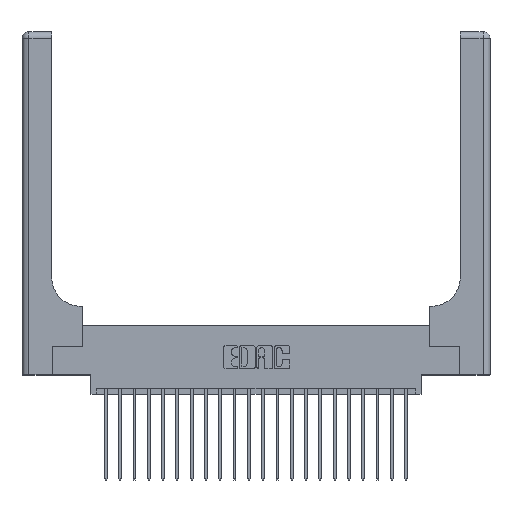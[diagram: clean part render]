
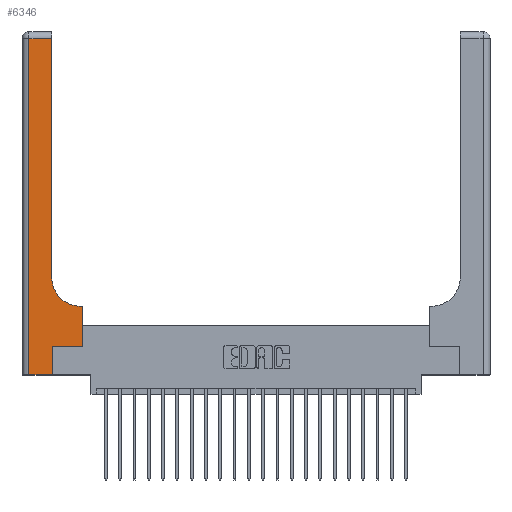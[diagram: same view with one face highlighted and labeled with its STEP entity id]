
A CAD part, top view. The second image highlights one B-rep face of the part: STEP entity #6346.
In plain terms, the highlighted planar face has unit normal (0, 0, 1).
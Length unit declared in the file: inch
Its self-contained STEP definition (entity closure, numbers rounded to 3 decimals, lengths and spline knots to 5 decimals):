
#209 = ORIENTED_EDGE ( 'NONE', *, *, #18631, .T. ) ;
#318 = CARTESIAN_POINT ( 'NONE',  ( 0.528, 0.6, 0.37 ) ) ;
#325 = VECTOR ( 'NONE', #9154, 39.37008 ) ;
#718 = CARTESIAN_POINT ( 'NONE',  ( 0., 3., 0.37 ) ) ;
#719 = ORIENTED_EDGE ( 'NONE', *, *, #10867, .T. ) ;
#832 = FACE_OUTER_BOUND ( 'NONE', #22626, .T. ) ;
#1018 = ORIENTED_EDGE ( 'NONE', *, *, #12879, .T. ) ;
#1352 = CARTESIAN_POINT ( 'NONE',  ( 0.265, 0.25, 0.37 ) ) ;
#1356 = LINE ( 'NONE', #21672, #8314 ) ;
#1602 = DIRECTION ( 'NONE',  ( 0., 1., 0. ) ) ;
#2286 = CARTESIAN_POINT ( 'NONE',  ( 0.528, 0.25, 0.37 ) ) ;
#2618 = VERTEX_POINT ( 'NONE', #15560 ) ;
#3192 = DIRECTION ( 'NONE',  ( 1., 0., 0. ) ) ;
#3220 = VECTOR ( 'NONE', #3192, 39.37008 ) ;
#3402 = DIRECTION ( 'NONE',  ( -1., 0., 0. ) ) ;
#3409 = VERTEX_POINT ( 'NONE', #13255 ) ;
#3488 = VERTEX_POINT ( 'NONE', #17016 ) ;
#3734 = VERTEX_POINT ( 'NONE', #8714 ) ;
#4235 = LINE ( 'NONE', #2286, #4493 ) ;
#4315 = CARTESIAN_POINT ( 'NONE',  ( 0., 0., 0.37 ) ) ;
#4481 = EDGE_CURVE ( 'NONE', #2618, #10803, #20533, .T. ) ;
#4493 = VECTOR ( 'NONE', #19701, 39.37008 ) ;
#4520 = VERTEX_POINT ( 'NONE', #17272 ) ;
#5045 = VECTOR ( 'NONE', #1602, 39.37008 ) ;
#5524 = EDGE_CURVE ( 'NONE', #3734, #18050, #4235, .T. ) ;
#6096 = VERTEX_POINT ( 'NONE', #16983 ) ;
#6346 = ADVANCED_FACE ( 'NONE', ( #832 ), #22198, .F. ) ;
#6915 = ORIENTED_EDGE ( 'NONE', *, *, #20098, .T. ) ;
#8314 = VECTOR ( 'NONE', #8965, 39.37008 ) ;
#8714 = CARTESIAN_POINT ( 'NONE',  ( 0.528, 0.25, 0.37 ) ) ;
#8965 = DIRECTION ( 'NONE',  ( -1., 0., 0. ) ) ;
#9154 = DIRECTION ( 'NONE',  ( 0., 1., 0. ) ) ;
#9383 = DIRECTION ( 'NONE',  ( 1., 0., 0. ) ) ;
#10392 = DIRECTION ( 'NONE',  ( 0., -1., 0. ) ) ;
#10803 = VERTEX_POINT ( 'NONE', #1352 ) ;
#10851 = CARTESIAN_POINT ( 'NONE',  ( 0.51, 0.6, 0.37 ) ) ;
#10867 = EDGE_CURVE ( 'NONE', #16644, #6096, #11961, .T. ) ;
#11488 = ORIENTED_EDGE ( 'NONE', *, *, #14473, .T. ) ;
#11646 = CARTESIAN_POINT ( 'NONE',  ( 0.265, 0., 0.37 ) ) ;
#11955 = LINE ( 'NONE', #18976, #3220 ) ;
#11961 = CIRCLE ( 'NONE', #13434, 0.25 ) ;
#12879 = EDGE_CURVE ( 'NONE', #18050, #16644, #1356, .T. ) ;
#13255 = CARTESIAN_POINT ( 'NONE',  ( 0.06, 0., 0.37 ) ) ;
#13434 = AXIS2_PLACEMENT_3D ( 'NONE', #18068, #14497, #14386 ) ;
#13739 = CARTESIAN_POINT ( 'NONE',  ( 0.06, 3., 0.37 ) ) ;
#14349 = LINE ( 'NONE', #21404, #325 ) ;
#14386 = DIRECTION ( 'NONE',  ( 1., 0., 0. ) ) ;
#14473 = EDGE_CURVE ( 'NONE', #10803, #3734, #11955, .T. ) ;
#14497 = DIRECTION ( 'NONE',  ( 0., 0., -1. ) ) ;
#14572 = LINE ( 'NONE', #4315, #20496 ) ;
#15344 = LINE ( 'NONE', #13739, #20985 ) ;
#15461 = VECTOR ( 'NONE', #3402, 39.37008 ) ;
#15560 = CARTESIAN_POINT ( 'NONE',  ( 0.265, 0., 0.37 ) ) ;
#15599 = LINE ( 'NONE', #19199, #15461 ) ;
#16644 = VERTEX_POINT ( 'NONE', #10851 ) ;
#16920 = ORIENTED_EDGE ( 'NONE', *, *, #18426, .T. ) ;
#16983 = CARTESIAN_POINT ( 'NONE',  ( 0.26, 0.85, 0.37 ) ) ;
#17016 = CARTESIAN_POINT ( 'NONE',  ( 0.06, 2.94, 0.37 ) ) ;
#17127 = ORIENTED_EDGE ( 'NONE', *, *, #22154, .T. ) ;
#17272 = CARTESIAN_POINT ( 'NONE',  ( 0.26, 2.94, 0.37 ) ) ;
#17976 = ORIENTED_EDGE ( 'NONE', *, *, #4481, .T. ) ;
#18050 = VERTEX_POINT ( 'NONE', #318 ) ;
#18068 = CARTESIAN_POINT ( 'NONE',  ( 0.51, 0.85, 0.37 ) ) ;
#18369 = DIRECTION ( 'NONE',  ( 0., 0., -1. ) ) ;
#18426 = EDGE_CURVE ( 'NONE', #6096, #4520, #14349, .T. ) ;
#18631 = EDGE_CURVE ( 'NONE', #3488, #3409, #15344, .T. ) ;
#18976 = CARTESIAN_POINT ( 'NONE',  ( 0.265, 0.25, 0.37 ) ) ;
#19199 = CARTESIAN_POINT ( 'NONE',  ( 0., 2.94, 0.37 ) ) ;
#19701 = DIRECTION ( 'NONE',  ( 0., 1., 0. ) ) ;
#20098 = EDGE_CURVE ( 'NONE', #4520, #3488, #15599, .T. ) ;
#20496 = VECTOR ( 'NONE', #9383, 39.37008 ) ;
#20533 = LINE ( 'NONE', #11646, #5045 ) ;
#20709 = AXIS2_PLACEMENT_3D ( 'NONE', #718, #18369, #20858 ) ;
#20805 = ORIENTED_EDGE ( 'NONE', *, *, #5524, .T. ) ;
#20858 = DIRECTION ( 'NONE',  ( -1., 0., 0. ) ) ;
#20985 = VECTOR ( 'NONE', #10392, 39.37008 ) ;
#21404 = CARTESIAN_POINT ( 'NONE',  ( 0.26, 3., 0.37 ) ) ;
#21672 = CARTESIAN_POINT ( 'NONE',  ( 0.26, 0.6, 0.37 ) ) ;
#22154 = EDGE_CURVE ( 'NONE', #3409, #2618, #14572, .T. ) ;
#22198 = PLANE ( 'NONE',  #20709 ) ;
#22626 = EDGE_LOOP ( 'NONE', ( #16920, #6915, #209, #17127, #17976, #11488, #20805, #1018, #719 ) ) ;
